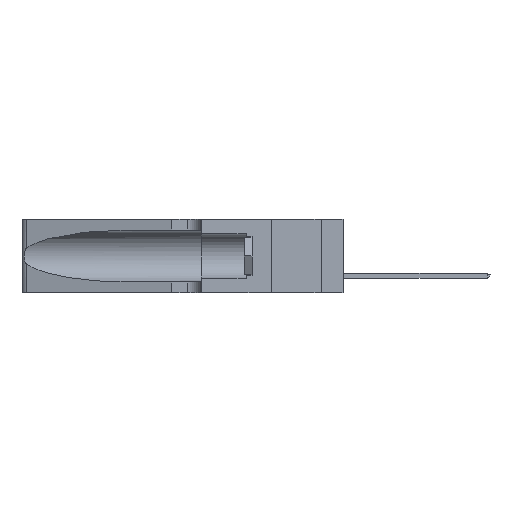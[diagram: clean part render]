
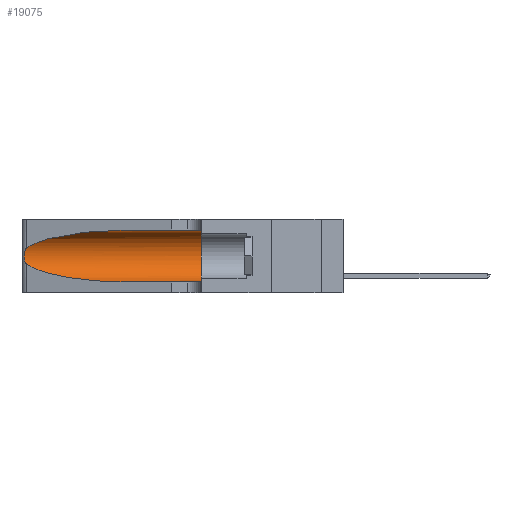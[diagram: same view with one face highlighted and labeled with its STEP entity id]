
A CAD part, left-side view. The second image highlights one B-rep face of the part: STEP entity #19075.
In plain terms, the highlighted cylindrical face has radius 3.308 mm (diameter 6.617 mm), a partial arc.
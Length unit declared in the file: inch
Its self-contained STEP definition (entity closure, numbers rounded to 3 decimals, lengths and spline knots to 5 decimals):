
#1160 = CARTESIAN_POINT ( 'NONE',  ( 0.2373, 1.15595, 0.28018 ) ) ;
#1969 = CARTESIAN_POINT ( 'NONE',  ( 0.1305, 0.35, 0.05475 ) ) ;
#2280 = EDGE_CURVE ( 'NONE', #30448, #5267, #25085, .T. ) ;
#3699 = ORIENTED_EDGE ( 'NONE', *, *, #2280, .F. ) ;
#3991 = CARTESIAN_POINT ( 'NONE',  ( 0.25555, 1.22994, 0.2215 ) ) ;
#4049 = ORIENTED_EDGE ( 'NONE', *, *, #17209, .T. ) ;
#4651 = CARTESIAN_POINT ( 'NONE',  ( 0.1305, 1.61858, 0.05475 ) ) ;
#4792 = FACE_OUTER_BOUND ( 'NONE', #10895, .T. ) ;
#5267 = VERTEX_POINT ( 'NONE', #32138 ) ;
#5551 = CARTESIAN_POINT ( 'NONE',  ( 0.25639, 1.23186, 0.15144 ) ) ;
#5633 = DIRECTION ( 'NONE',  ( 0., -1., 0. ) ) ;
#6182 = EDGE_CURVE ( 'NONE', #30448, #38005, #29260, .T. ) ;
#6548 = CARTESIAN_POINT ( 'NONE',  ( 0.2373, 1.15595, 0.08982 ) ) ;
#7726 = CARTESIAN_POINT ( 'NONE',  ( 0.25487, 1.22718, 0.22369 ) ) ;
#8600 = CARTESIAN_POINT ( 'NONE',  ( 0.26075, 1.23896, 0.19203 ) ) ;
#10027 = DIRECTION ( 'NONE',  ( 0., 0., -1. ) ) ;
#10237 = CARTESIAN_POINT ( 'NONE',  ( 0.18966, 0.96281, 0.05475 ) ) ;
#10895 = EDGE_LOOP ( 'NONE', ( #14651, #15348, #41394, #4049, #26396, #3699 ) ) ;
#11254 = EDGE_CURVE ( 'NONE', #5267, #33420, #35635, .T. ) ;
#11792 = CARTESIAN_POINT ( 'NONE',  ( 0.25487, 1.22718, 0.22369 ) ) ;
#11900 = AXIS2_PLACEMENT_3D ( 'NONE', #28033, #31680, #10027 ) ;
#12022 = CARTESIAN_POINT ( 'NONE',  ( 0.1305, 0.72297, 0.31525 ) ) ;
#12208 = CARTESIAN_POINT ( 'NONE',  ( 0.25487, 1.22718, 0.14631 ) ) ;
#12749 = CARTESIAN_POINT ( 'NONE',  ( 0.25555, 1.22993, 0.14849 ) ) ;
#14651 = ORIENTED_EDGE ( 'NONE', *, *, #6182, .T. ) ;
#15348 = ORIENTED_EDGE ( 'NONE', *, *, #18064, .T. ) ;
#15743 = CARTESIAN_POINT ( 'NONE',  ( 0.26075, 1.23896, 0.178 ) ) ;
#15960 = DIRECTION ( 'NONE',  ( 0., -1., 0. ) ) ;
#16062 = CARTESIAN_POINT ( 'NONE',  ( 0.25856, 1.23593, 0.16098 ) ) ;
#17209 = EDGE_CURVE ( 'NONE', #18893, #33420, #42471, .T. ) ;
#18064 = EDGE_CURVE ( 'NONE', #38005, #30708, #44916, .T. ) ;
#18893 = VERTEX_POINT ( 'NONE', #20179 ) ;
#19075 = ADVANCED_FACE ( 'NONE', ( #4792 ), #46814, .F. ) ;
#19096 =( BOUNDED_CURVE ( )  B_SPLINE_CURVE ( 3, ( #31099, #6548, #10237, #35543 ),
 .UNSPECIFIED., .F., .T. ) 
 B_SPLINE_CURVE_WITH_KNOTS ( ( 4, 4 ),
 ( 3.44316, 4.71239 ),
 .UNSPECIFIED. ) 
 CURVE ( )  GEOMETRIC_REPRESENTATION_ITEM ( )  RATIONAL_B_SPLINE_CURVE ( ( 1., 0.87, 0.87, 1. ) ) 
 REPRESENTATION_ITEM ( '' )  );
#20179 = CARTESIAN_POINT ( 'NONE',  ( 0.1305, 0.72297, 0.05475 ) ) ;
#21255 = CARTESIAN_POINT ( 'NONE',  ( 0.1305, 0.35, 0.185 ) ) ;
#22670 = CARTESIAN_POINT ( 'NONE',  ( 0.25854, 1.2359, 0.20912 ) ) ;
#23571 = CARTESIAN_POINT ( 'NONE',  ( 0.1305, 1.61858, 0.31525 ) ) ;
#24575 = DIRECTION ( 'NONE',  ( 0., 0., 1. ) ) ;
#25085 = LINE ( 'NONE', #23571, #37456 ) ;
#25674 = CARTESIAN_POINT ( 'NONE',  ( 0.25487, 1.22718, 0.22369 ) ) ;
#26396 = ORIENTED_EDGE ( 'NONE', *, *, #11254, .F. ) ;
#26786 = CARTESIAN_POINT ( 'NONE',  ( 0.26017, 1.23833, 0.17102 ) ) ;
#27748 = CARTESIAN_POINT ( 'NONE',  ( 0.25789, 1.23486, 0.15765 ) ) ;
#28033 = CARTESIAN_POINT ( 'NONE',  ( 0.1305, 1.61858, 0.185 ) ) ;
#29260 =( BOUNDED_CURVE ( )  B_SPLINE_CURVE ( 3, ( #12022, #40953, #1160, #7726 ),
 .UNSPECIFIED., .F., .F. ) 
 B_SPLINE_CURVE_WITH_KNOTS ( ( 4, 4 ),
 ( 1.5708, 2.84003 ),
 .UNSPECIFIED. ) 
 CURVE ( )  GEOMETRIC_REPRESENTATION_ITEM ( )  RATIONAL_B_SPLINE_CURVE ( ( 1., 0.87, 0.87, 1. ) ) 
 REPRESENTATION_ITEM ( '' )  );
#30448 = VERTEX_POINT ( 'NONE', #31930 ) ;
#30708 = VERTEX_POINT ( 'NONE', #12208 ) ;
#31099 = CARTESIAN_POINT ( 'NONE',  ( 0.25487, 1.22718, 0.14631 ) ) ;
#31680 = DIRECTION ( 'NONE',  ( 0., -1., 0. ) ) ;
#31825 = DIRECTION ( 'NONE',  ( 0., 1., 0. ) ) ;
#31930 = CARTESIAN_POINT ( 'NONE',  ( 0.1305, 0.72297, 0.31525 ) ) ;
#32138 = CARTESIAN_POINT ( 'NONE',  ( 0.1305, 0.35, 0.31525 ) ) ;
#32785 = VECTOR ( 'NONE', #15960, 39.37008 ) ;
#33098 = CARTESIAN_POINT ( 'NONE',  ( 0.25639, 1.23184, 0.21858 ) ) ;
#33420 = VERTEX_POINT ( 'NONE', #1969 ) ;
#33618 = AXIS2_PLACEMENT_3D ( 'NONE', #21255, #31825, #24575 ) ;
#33734 = CARTESIAN_POINT ( 'NONE',  ( 0.26018, 1.23835, 0.19895 ) ) ;
#35543 = CARTESIAN_POINT ( 'NONE',  ( 0.1305, 0.72297, 0.05475 ) ) ;
#35635 = CIRCLE ( 'NONE', #33618, 0.13025 ) ;
#36770 = CARTESIAN_POINT ( 'NONE',  ( 0.25787, 1.23484, 0.2124 ) ) ;
#37456 = VECTOR ( 'NONE', #5633, 39.37008 ) ;
#38005 = VERTEX_POINT ( 'NONE', #25674 ) ;
#38329 = CARTESIAN_POINT ( 'NONE',  ( 0.25487, 1.22718, 0.14631 ) ) ;
#40953 = CARTESIAN_POINT ( 'NONE',  ( 0.18966, 0.96281, 0.31525 ) ) ;
#41394 = ORIENTED_EDGE ( 'NONE', *, *, #42201, .T. ) ;
#42201 = EDGE_CURVE ( 'NONE', #30708, #18893, #19096, .T. ) ;
#42471 = LINE ( 'NONE', #4651, #32785 ) ;
#44916 = B_SPLINE_CURVE_WITH_KNOTS ( 'NONE', 3,
 ( #11792, #3991, #33098, #36770, #22670, #33734, #8600, #15743, #26786, #16062, #27748, #5551, #12749, #38329 ),
 .UNSPECIFIED., .F., .F.,
 ( 4, 2, 2, 2, 2, 2, 4 ),
 ( 0., 0.00027, 0.00053, 0.00107, 0.0016, 0.00187, 0.00214 ),
 .UNSPECIFIED. ) ;
#46814 = CYLINDRICAL_SURFACE ( 'NONE', #11900, 0.13025 ) ;
